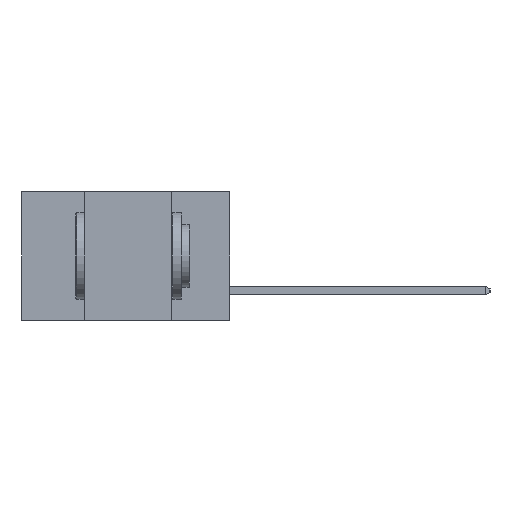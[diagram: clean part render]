
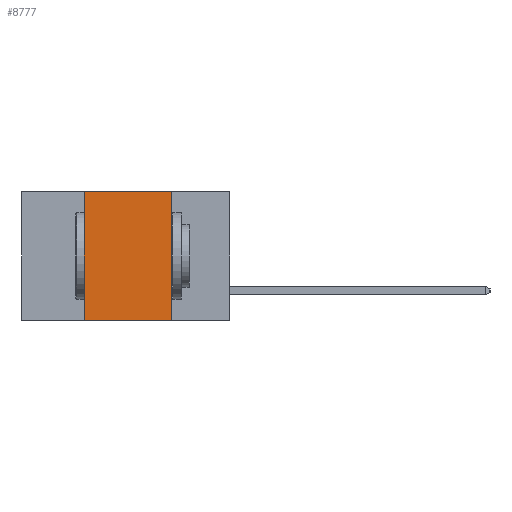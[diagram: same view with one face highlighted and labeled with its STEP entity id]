
A CAD part, left-side view. The second image highlights one B-rep face of the part: STEP entity #8777.
In plain terms, the highlighted planar face has unit normal (-1, 0, 0).
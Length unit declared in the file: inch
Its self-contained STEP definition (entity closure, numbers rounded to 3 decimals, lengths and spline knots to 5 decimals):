
#1469 = CARTESIAN_POINT ( 'NONE',  ( 0., 0.6, 0. ) ) ;
#1989 = CARTESIAN_POINT ( 'NONE',  ( 0., 0.17, 0. ) ) ;
#2098 = ORIENTED_EDGE ( 'NONE', *, *, #17847, .T. ) ;
#4090 = DIRECTION ( 'NONE',  ( 0., 0., -1. ) ) ;
#5676 = LINE ( 'NONE', #8039, #10011 ) ;
#6300 = VERTEX_POINT ( 'NONE', #13751 ) ;
#8039 = CARTESIAN_POINT ( 'NONE',  ( 0., 0.42, -0.37 ) ) ;
#8432 = VECTOR ( 'NONE', #11811, 39.37008 ) ;
#8777 = ADVANCED_FACE ( 'NONE', ( #20117 ), #25677, .F. ) ;
#10011 = VECTOR ( 'NONE', #18604, 39.37008 ) ;
#11811 = DIRECTION ( 'NONE',  ( 0., -1., 0. ) ) ;
#12069 = ORIENTED_EDGE ( 'NONE', *, *, #24587, .F. ) ;
#13751 = CARTESIAN_POINT ( 'NONE',  ( 0., 0.42, -0.37 ) ) ;
#14737 = DIRECTION ( 'NONE',  ( 0., -1., 0. ) ) ;
#15626 = VECTOR ( 'NONE', #4090, 39.37008 ) ;
#17218 = AXIS2_PLACEMENT_3D ( 'NONE', #25627, #25547, #25540 ) ;
#17847 = EDGE_CURVE ( 'NONE', #6300, #24487, #24910, .T. ) ;
#18604 = DIRECTION ( 'NONE',  ( 0., 0., 1. ) ) ;
#18811 = CARTESIAN_POINT ( 'NONE',  ( 0., 0.17, -0.37 ) ) ;
#18937 = VERTEX_POINT ( 'NONE', #21826 ) ;
#19222 = EDGE_CURVE ( 'NONE', #6300, #18937, #5676, .T. ) ;
#19836 = EDGE_LOOP ( 'NONE', ( #21800, #12069, #23025, #2098 ) ) ;
#20117 = FACE_OUTER_BOUND ( 'NONE', #19836, .T. ) ;
#20300 = VERTEX_POINT ( 'NONE', #1989 ) ;
#21093 = LINE ( 'NONE', #18811, #15626 ) ;
#21800 = ORIENTED_EDGE ( 'NONE', *, *, #25967, .F. ) ;
#21826 = CARTESIAN_POINT ( 'NONE',  ( 0., 0.42, 0. ) ) ;
#22127 = CARTESIAN_POINT ( 'NONE',  ( 0., 0.6, -0.37 ) ) ;
#22193 = CARTESIAN_POINT ( 'NONE',  ( 0., 0.17, -0.37 ) ) ;
#23025 = ORIENTED_EDGE ( 'NONE', *, *, #19222, .F. ) ;
#23027 = VECTOR ( 'NONE', #14737, 39.37008 ) ;
#23655 = LINE ( 'NONE', #1469, #23027 ) ;
#24487 = VERTEX_POINT ( 'NONE', #22193 ) ;
#24587 = EDGE_CURVE ( 'NONE', #18937, #20300, #23655, .T. ) ;
#24910 = LINE ( 'NONE', #22127, #8432 ) ;
#25540 = DIRECTION ( 'NONE',  ( 0., 0., -1. ) ) ;
#25547 = DIRECTION ( 'NONE',  ( 1., 0., 0. ) ) ;
#25627 = CARTESIAN_POINT ( 'NONE',  ( 0., 0.6, 0. ) ) ;
#25677 = PLANE ( 'NONE',  #17218 ) ;
#25967 = EDGE_CURVE ( 'NONE', #20300, #24487, #21093, .T. ) ;
